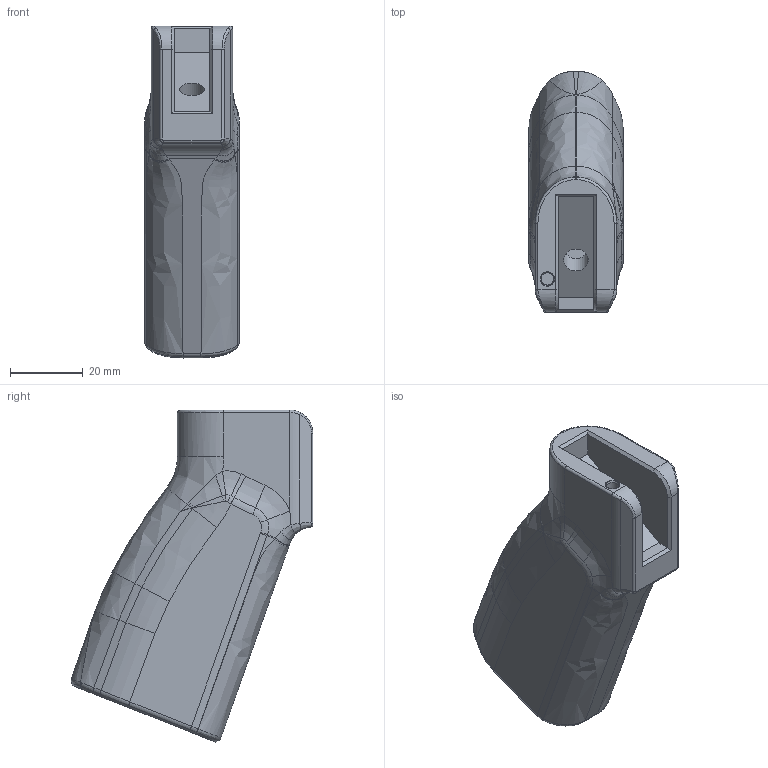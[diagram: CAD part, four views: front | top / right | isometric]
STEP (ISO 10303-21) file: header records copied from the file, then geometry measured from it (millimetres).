
FILE_DESCRIPTION(/* description */ (''),/* implementation_level */ '2;1');
FILE_NAME(/* name */ 'Lil Chonk.step',/* time_stamp */ '2021-05-07T10:03:29-04:00',/* author */ (''),/* organization */ (''),/* preprocessor_version */ 'ST-DEVELOPER v18.1',/* originating_system */ 'Autodesk Translation Framework v10.6.0.1341',/* authorisation */ '');
FILE_SCHEMA (('AUTOMOTIVE_DESIGN { 1 0 10303 214 3 1 1 }'));
Length unit declared in the file: millimetre
Products named in the file (1): Lil Chonk
Bounding box: 25.93 x 66.4 x 91.21 mm (x, y, z)
Volume: 37813.2 mm3; surface area: 18791.2 mm2
Topology: 1 solids, 3 shells, 416 faces, 1002 edges, 580 vertices
Faces by surface type: bspline 288, cylinder 58, plane 43, torus 22, cone 3, sphere 2
Full cylindrical faces by diameter (mm): 3.4 x1, 6.8 x1
Entity records: 18887 total; most frequent: CARTESIAN_POINT 11096, ORIENTED_EDGE 1968, EDGE_CURVE 984, DIRECTION 983, VERTEX_POINT 580, B_SPLINE_CURVE_WITH_KNOTS 525, EDGE_LOOP 424, FACE_OUTER_BOUND 416
